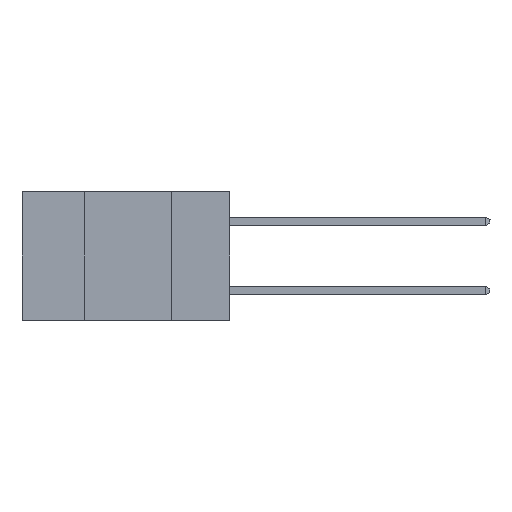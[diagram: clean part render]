
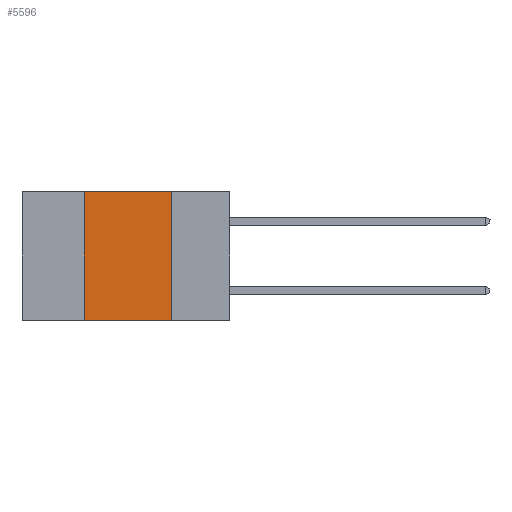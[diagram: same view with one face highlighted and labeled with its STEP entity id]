
A CAD part, left-side view. The second image highlights one B-rep face of the part: STEP entity #5596.
In plain terms, the highlighted planar face has unit normal (-1, 0, 0).
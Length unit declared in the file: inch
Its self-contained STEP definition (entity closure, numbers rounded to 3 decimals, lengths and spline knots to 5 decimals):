
#763 = VERTEX_POINT ( 'NONE', #1391 ) ;
#838 = DIRECTION ( 'NONE',  ( 0., 0., 1. ) ) ;
#1391 = CARTESIAN_POINT ( 'NONE',  ( 0., 0.17, 0. ) ) ;
#1515 = CARTESIAN_POINT ( 'NONE',  ( 0., 0.17, -0.37 ) ) ;
#1898 = CARTESIAN_POINT ( 'NONE',  ( 0., 0.42, 0. ) ) ;
#2177 = VERTEX_POINT ( 'NONE', #9514 ) ;
#2422 = FACE_OUTER_BOUND ( 'NONE', #12460, .T. ) ;
#2691 = EDGE_CURVE ( 'NONE', #14783, #763, #4101, .T. ) ;
#2767 = DIRECTION ( 'NONE',  ( 0., -1., 0. ) ) ;
#3309 = EDGE_CURVE ( 'NONE', #763, #15661, #14920, .T. ) ;
#3839 = DIRECTION ( 'NONE',  ( 1., 0., 0. ) ) ;
#3841 = CARTESIAN_POINT ( 'NONE',  ( 0., 0.6, 0. ) ) ;
#4038 = EDGE_CURVE ( 'NONE', #2177, #15661, #5240, .T. ) ;
#4101 = LINE ( 'NONE', #3841, #10178 ) ;
#4291 = VECTOR ( 'NONE', #9466, 39.37008 ) ;
#4458 = EDGE_CURVE ( 'NONE', #2177, #14783, #5047, .T. ) ;
#5047 = LINE ( 'NONE', #10437, #8543 ) ;
#5240 = LINE ( 'NONE', #12210, #4291 ) ;
#5596 = ADVANCED_FACE ( 'NONE', ( #2422 ), #14246, .F. ) ;
#6209 = VECTOR ( 'NONE', #12185, 39.37008 ) ;
#8000 = AXIS2_PLACEMENT_3D ( 'NONE', #15920, #3839, #14592 ) ;
#8543 = VECTOR ( 'NONE', #838, 39.37008 ) ;
#9466 = DIRECTION ( 'NONE',  ( 0., -1., 0. ) ) ;
#9514 = CARTESIAN_POINT ( 'NONE',  ( 0., 0.42, -0.37 ) ) ;
#10178 = VECTOR ( 'NONE', #2767, 39.37008 ) ;
#10413 = ORIENTED_EDGE ( 'NONE', *, *, #4038, .T. ) ;
#10437 = CARTESIAN_POINT ( 'NONE',  ( 0., 0.42, -0.37 ) ) ;
#12116 = ORIENTED_EDGE ( 'NONE', *, *, #3309, .F. ) ;
#12185 = DIRECTION ( 'NONE',  ( 0., 0., -1. ) ) ;
#12210 = CARTESIAN_POINT ( 'NONE',  ( 0., 0.6, -0.37 ) ) ;
#12460 = EDGE_LOOP ( 'NONE', ( #12116, #14431, #14665, #10413 ) ) ;
#14246 = PLANE ( 'NONE',  #8000 ) ;
#14431 = ORIENTED_EDGE ( 'NONE', *, *, #2691, .F. ) ;
#14592 = DIRECTION ( 'NONE',  ( 0., 0., -1. ) ) ;
#14665 = ORIENTED_EDGE ( 'NONE', *, *, #4458, .F. ) ;
#14783 = VERTEX_POINT ( 'NONE', #1898 ) ;
#14920 = LINE ( 'NONE', #1515, #6209 ) ;
#15661 = VERTEX_POINT ( 'NONE', #17420 ) ;
#15920 = CARTESIAN_POINT ( 'NONE',  ( 0., 0.6, 0. ) ) ;
#17420 = CARTESIAN_POINT ( 'NONE',  ( 0., 0.17, -0.37 ) ) ;
